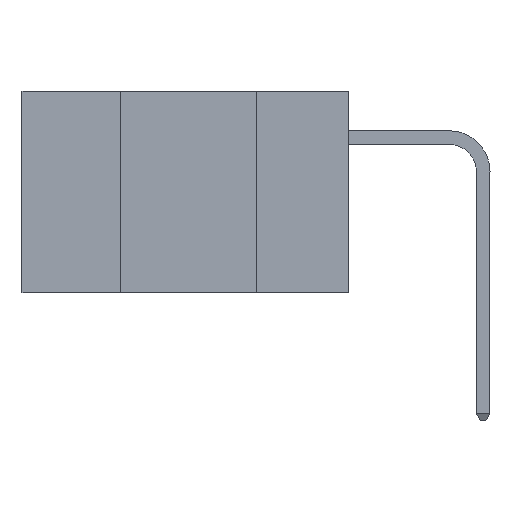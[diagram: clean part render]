
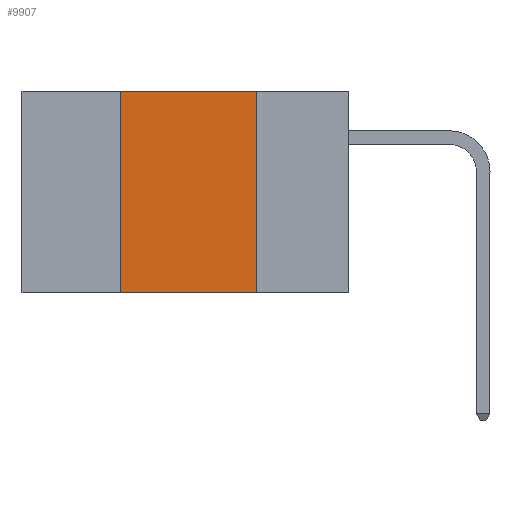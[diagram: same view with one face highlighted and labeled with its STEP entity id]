
A CAD part, left-side view. The second image highlights one B-rep face of the part: STEP entity #9907.
In plain terms, the highlighted planar face has unit normal (-1, 0, 0).
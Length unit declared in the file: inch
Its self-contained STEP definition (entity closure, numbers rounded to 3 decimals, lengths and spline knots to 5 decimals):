
#9 = EDGE_CURVE ( 'NONE', #737, #1028, #7071, .T. ) ;
#19 = EDGE_CURVE ( 'NONE', #737, #517, #6514, .T. ) ;
#330 = DIRECTION ( 'NONE',  ( 1., 0., 0. ) ) ;
#517 = VERTEX_POINT ( 'NONE', #5595 ) ;
#696 = DIRECTION ( 'NONE',  ( 0., 0., 1. ) ) ;
#737 = VERTEX_POINT ( 'NONE', #1908 ) ;
#946 = VECTOR ( 'NONE', #8277, 39.37008 ) ;
#1028 = VERTEX_POINT ( 'NONE', #6815 ) ;
#1180 = LINE ( 'NONE', #5829, #946 ) ;
#1292 = ORIENTED_EDGE ( 'NONE', *, *, #9, .F. ) ;
#1908 = CARTESIAN_POINT ( 'NONE',  ( 0., 0.42, -0.37 ) ) ;
#2075 = DIRECTION ( 'NONE',  ( 0., -1., 0. ) ) ;
#3449 = CARTESIAN_POINT ( 'NONE',  ( 0., 0.6, -0.37 ) ) ;
#3813 = DIRECTION ( 'NONE',  ( 0., -1., 0. ) ) ;
#3951 = ORIENTED_EDGE ( 'NONE', *, *, #19, .T. ) ;
#5595 = CARTESIAN_POINT ( 'NONE',  ( 0., 0.17, -0.37 ) ) ;
#5741 = VERTEX_POINT ( 'NONE', #6545 ) ;
#5829 = CARTESIAN_POINT ( 'NONE',  ( 0., 0.17, 0. ) ) ;
#6430 = VECTOR ( 'NONE', #3813, 39.37008 ) ;
#6514 = LINE ( 'NONE', #3449, #6430 ) ;
#6545 = CARTESIAN_POINT ( 'NONE',  ( 0., 0.17, 0. ) ) ;
#6815 = CARTESIAN_POINT ( 'NONE',  ( 0., 0.42, 0. ) ) ;
#6865 = CARTESIAN_POINT ( 'NONE',  ( 0., 0.6, 0. ) ) ;
#6906 = DIRECTION ( 'NONE',  ( 0., 0., -1. ) ) ;
#7071 = LINE ( 'NONE', #7992, #9811 ) ;
#7430 = VECTOR ( 'NONE', #2075, 39.37008 ) ;
#7580 = EDGE_LOOP ( 'NONE', ( #7645, #9452, #1292, #3951 ) ) ;
#7645 = ORIENTED_EDGE ( 'NONE', *, *, #7847, .F. ) ;
#7847 = EDGE_CURVE ( 'NONE', #5741, #517, #1180, .T. ) ;
#7892 = LINE ( 'NONE', #8290, #7430 ) ;
#7992 = CARTESIAN_POINT ( 'NONE',  ( 0., 0.42, 0. ) ) ;
#8277 = DIRECTION ( 'NONE',  ( 0., 0., -1. ) ) ;
#8290 = CARTESIAN_POINT ( 'NONE',  ( 0., 0.6, 0. ) ) ;
#8418 = FACE_OUTER_BOUND ( 'NONE', #7580, .T. ) ;
#9183 = PLANE ( 'NONE',  #9847 ) ;
#9452 = ORIENTED_EDGE ( 'NONE', *, *, #10500, .F. ) ;
#9811 = VECTOR ( 'NONE', #696, 39.37008 ) ;
#9847 = AXIS2_PLACEMENT_3D ( 'NONE', #6865, #330, #6906 ) ;
#9907 = ADVANCED_FACE ( 'NONE', ( #8418 ), #9183, .F. ) ;
#10500 = EDGE_CURVE ( 'NONE', #1028, #5741, #7892, .T. ) ;
